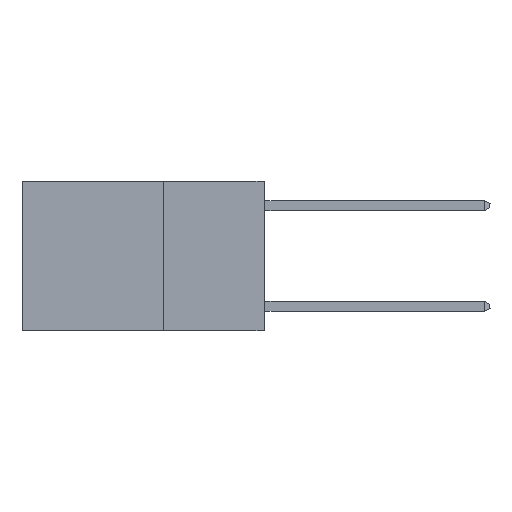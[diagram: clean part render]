
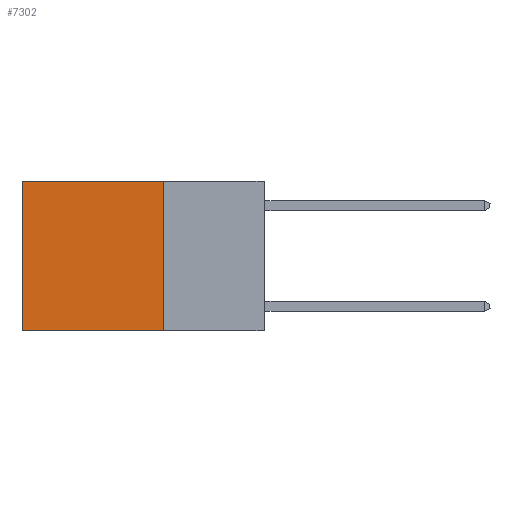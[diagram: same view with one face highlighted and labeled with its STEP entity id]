
A CAD part, left-side view. The second image highlights one B-rep face of the part: STEP entity #7302.
In plain terms, the highlighted planar face has unit normal (-1, 0, 0).
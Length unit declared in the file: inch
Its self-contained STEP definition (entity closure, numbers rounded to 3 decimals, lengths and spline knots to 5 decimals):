
#843 = VECTOR ( 'NONE', #6670, 39.37008 ) ;
#991 = EDGE_CURVE ( 'NONE', #7020, #3231, #11154, .T. ) ;
#1780 = VERTEX_POINT ( 'NONE', #12768 ) ;
#1831 = AXIS2_PLACEMENT_3D ( 'NONE', #7350, #1959, #11644 ) ;
#1959 = DIRECTION ( 'NONE',  ( 1., 0., 0. ) ) ;
#2712 = DIRECTION ( 'NONE',  ( 0., 0., -1. ) ) ;
#3231 = VERTEX_POINT ( 'NONE', #7754 ) ;
#3711 = EDGE_LOOP ( 'NONE', ( #8056, #8220, #7672, #8905 ) ) ;
#4425 = EDGE_CURVE ( 'NONE', #1780, #8108, #11372, .T. ) ;
#4452 = LINE ( 'NONE', #7752, #8328 ) ;
#5361 = EDGE_CURVE ( 'NONE', #8108, #3231, #5958, .T. ) ;
#5958 = LINE ( 'NONE', #9319, #11434 ) ;
#6602 = CARTESIAN_POINT ( 'NONE',  ( 0.2625, 0.6, 0. ) ) ;
#6670 = DIRECTION ( 'NONE',  ( 0., 0., -1. ) ) ;
#6690 = VECTOR ( 'NONE', #2712, 39.37008 ) ;
#7020 = VERTEX_POINT ( 'NONE', #9900 ) ;
#7157 = DIRECTION ( 'NONE',  ( 0., 1., 0. ) ) ;
#7302 = ADVANCED_FACE ( 'NONE', ( #9379 ), #7490, .F. ) ;
#7350 = CARTESIAN_POINT ( 'NONE',  ( 0.2625, 0.25, 0. ) ) ;
#7388 = CARTESIAN_POINT ( 'NONE',  ( 0.2625, 0.25, -0.37 ) ) ;
#7490 = PLANE ( 'NONE',  #1831 ) ;
#7672 = ORIENTED_EDGE ( 'NONE', *, *, #4425, .F. ) ;
#7752 = CARTESIAN_POINT ( 'NONE',  ( 0.2625, 0.25, 0. ) ) ;
#7754 = CARTESIAN_POINT ( 'NONE',  ( 0.2625, 0.6, -0.37 ) ) ;
#7829 = EDGE_CURVE ( 'NONE', #1780, #7020, #4452, .T. ) ;
#8056 = ORIENTED_EDGE ( 'NONE', *, *, #991, .T. ) ;
#8108 = VERTEX_POINT ( 'NONE', #7388 ) ;
#8220 = ORIENTED_EDGE ( 'NONE', *, *, #5361, .F. ) ;
#8328 = VECTOR ( 'NONE', #12909, 39.37008 ) ;
#8905 = ORIENTED_EDGE ( 'NONE', *, *, #7829, .T. ) ;
#9319 = CARTESIAN_POINT ( 'NONE',  ( 0.2625, 0.25, -0.37 ) ) ;
#9379 = FACE_OUTER_BOUND ( 'NONE', #3711, .T. ) ;
#9900 = CARTESIAN_POINT ( 'NONE',  ( 0.2625, 0.6, 0. ) ) ;
#11154 = LINE ( 'NONE', #6602, #843 ) ;
#11372 = LINE ( 'NONE', #12222, #6690 ) ;
#11434 = VECTOR ( 'NONE', #7157, 39.37008 ) ;
#11644 = DIRECTION ( 'NONE',  ( 0., 0., -1. ) ) ;
#12222 = CARTESIAN_POINT ( 'NONE',  ( 0.2625, 0.25, 0. ) ) ;
#12768 = CARTESIAN_POINT ( 'NONE',  ( 0.2625, 0.25, 0. ) ) ;
#12909 = DIRECTION ( 'NONE',  ( 0., 1., 0. ) ) ;
